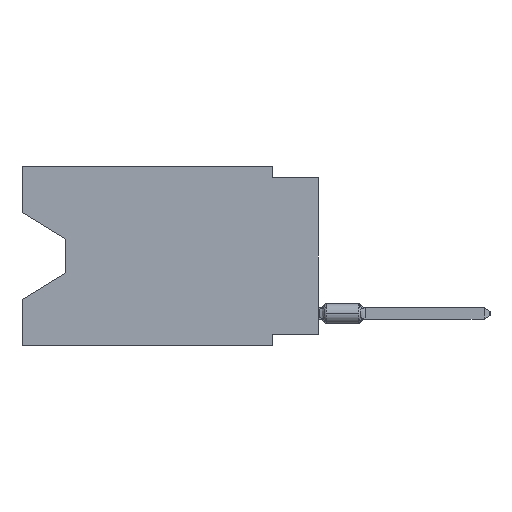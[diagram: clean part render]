
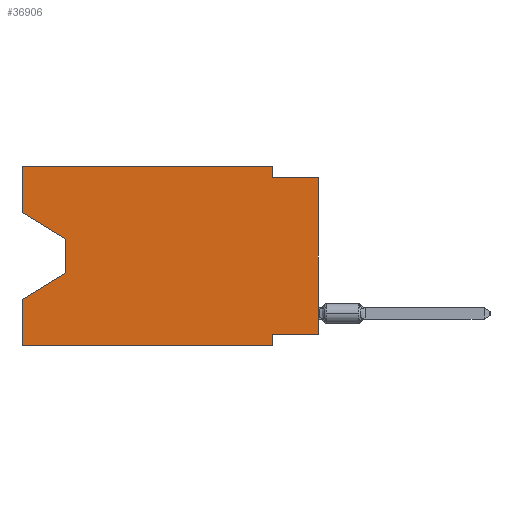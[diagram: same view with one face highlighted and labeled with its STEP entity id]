
A CAD part, left-side view. The second image highlights one B-rep face of the part: STEP entity #36906.
In plain terms, the highlighted planar face has unit normal (-1, 0, 0).
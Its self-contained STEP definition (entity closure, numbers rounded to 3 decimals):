
#1570 = ORIENTED_EDGE ( 'NONE', *, *, #34672, .F. ) ;
#1646 = CARTESIAN_POINT ( 'NONE',  ( 0., 16.383, 0. ) ) ;
#3146 = ORIENTED_EDGE ( 'NONE', *, *, #23481, .T. ) ;
#3249 = VECTOR ( 'NONE', #10510, 1000. ) ;
#3300 = CARTESIAN_POINT ( 'NONE',  ( 0., 16.383, -9.906 ) ) ;
#3720 = EDGE_CURVE ( 'NONE', #20055, #40407, #57582, .T. ) ;
#4301 = VERTEX_POINT ( 'NONE', #23348 ) ;
#4450 = CARTESIAN_POINT ( 'NONE',  ( 0., 0., -0.635 ) ) ;
#5240 = LINE ( 'NONE', #55700, #3249 ) ;
#5429 = CARTESIAN_POINT ( 'NONE',  ( 0., 2.54, -9.906 ) ) ;
#5473 = VECTOR ( 'NONE', #40983, 1000. ) ;
#6020 = VECTOR ( 'NONE', #51335, 1000. ) ;
#6224 = VERTEX_POINT ( 'NONE', #4450 ) ;
#7016 = CARTESIAN_POINT ( 'NONE',  ( 0., 2.54, 0. ) ) ;
#7504 = CARTESIAN_POINT ( 'NONE',  ( 0., 13.97, -5.893 ) ) ;
#8393 = CARTESIAN_POINT ( 'NONE',  ( 0., 2.54, 0. ) ) ;
#9225 = CARTESIAN_POINT ( 'NONE',  ( 0., 16.383, -7.36 ) ) ;
#10033 = FACE_OUTER_BOUND ( 'NONE', #16838, .T. ) ;
#10403 = DIRECTION ( 'NONE',  ( 0., 0., -1. ) ) ;
#10510 = DIRECTION ( 'NONE',  ( 0., 1., 0. ) ) ;
#10766 = EDGE_CURVE ( 'NONE', #26758, #56747, #36832, .T. ) ;
#11138 = PLANE ( 'NONE',  #38106 ) ;
#11255 = EDGE_CURVE ( 'NONE', #62127, #6224, #18677, .T. ) ;
#13391 = LINE ( 'NONE', #7016, #31921 ) ;
#14944 = LINE ( 'NONE', #3300, #43473 ) ;
#14978 = ORIENTED_EDGE ( 'NONE', *, *, #29583, .T. ) ;
#15608 = CARTESIAN_POINT ( 'NONE',  ( 0., 0., -9.271 ) ) ;
#16241 = VECTOR ( 'NONE', #24586, 1000. ) ;
#16386 = VECTOR ( 'NONE', #64615, 1000. ) ;
#16838 = EDGE_LOOP ( 'NONE', ( #51085, #14978, #63160, #18226, #58451, #65640, #35333, #3146, #51564, #34898, #33707, #1570 ) ) ;
#17080 = EDGE_CURVE ( 'NONE', #40627, #57894, #56996, .T. ) ;
#18226 = ORIENTED_EDGE ( 'NONE', *, *, #32633, .F. ) ;
#18677 = LINE ( 'NONE', #41646, #16386 ) ;
#19133 = CARTESIAN_POINT ( 'NONE',  ( 0., 13.97, -4.013 ) ) ;
#19805 = CARTESIAN_POINT ( 'NONE',  ( 0., 16.383, 0. ) ) ;
#20055 = VERTEX_POINT ( 'NONE', #38810 ) ;
#20527 = VECTOR ( 'NONE', #57102, 1000. ) ;
#23348 = CARTESIAN_POINT ( 'NONE',  ( 0., 16.383, -9.906 ) ) ;
#23481 = EDGE_CURVE ( 'NONE', #73886, #6224, #68775, .T. ) ;
#24586 = DIRECTION ( 'NONE',  ( 0., 0., 1. ) ) ;
#24704 = VECTOR ( 'NONE', #47370, 1000. ) ;
#26440 = VECTOR ( 'NONE', #57715, 1000. ) ;
#26758 = VERTEX_POINT ( 'NONE', #62379 ) ;
#29583 = EDGE_CURVE ( 'NONE', #56747, #20055, #70055, .T. ) ;
#29831 = LINE ( 'NONE', #46038, #26440 ) ;
#29864 = LINE ( 'NONE', #1646, #16241 ) ;
#30479 = EDGE_CURVE ( 'NONE', #39617, #62127, #13391, .T. ) ;
#30658 = VECTOR ( 'NONE', #57644, 1000. ) ;
#31921 = VECTOR ( 'NONE', #35970, 1000. ) ;
#32633 = EDGE_CURVE ( 'NONE', #4301, #40407, #42075, .T. ) ;
#33707 = ORIENTED_EDGE ( 'NONE', *, *, #39507, .F. ) ;
#34672 = EDGE_CURVE ( 'NONE', #26758, #59126, #29864, .T. ) ;
#34898 = ORIENTED_EDGE ( 'NONE', *, *, #30479, .F. ) ;
#35333 = ORIENTED_EDGE ( 'NONE', *, *, #70067, .F. ) ;
#35970 = DIRECTION ( 'NONE',  ( 0., 0., -1. ) ) ;
#36832 = LINE ( 'NONE', #42860, #24704 ) ;
#36906 = ADVANCED_FACE ( 'NONE', ( #10033 ), #11138, .F. ) ;
#38106 = AXIS2_PLACEMENT_3D ( 'NONE', #38989, #61964, #10403 ) ;
#38810 = CARTESIAN_POINT ( 'NONE',  ( 0., 13.97, -5.893 ) ) ;
#38989 = CARTESIAN_POINT ( 'NONE',  ( 0., 16.383, 0. ) ) ;
#39507 = EDGE_CURVE ( 'NONE', #59126, #39617, #29831, .T. ) ;
#39617 = VERTEX_POINT ( 'NONE', #8393 ) ;
#40407 = VERTEX_POINT ( 'NONE', #9225 ) ;
#40627 = VERTEX_POINT ( 'NONE', #44940 ) ;
#40875 = CARTESIAN_POINT ( 'NONE',  ( 0., 0., 0. ) ) ;
#40983 = DIRECTION ( 'NONE',  ( 0., 0.855, -0.519 ) ) ;
#41646 = CARTESIAN_POINT ( 'NONE',  ( 0., 0., -0.635 ) ) ;
#42075 = LINE ( 'NONE', #65052, #70453 ) ;
#42860 = CARTESIAN_POINT ( 'NONE',  ( 0., 16.383, -2.546 ) ) ;
#43473 = VECTOR ( 'NONE', #49193, 1000. ) ;
#44940 = CARTESIAN_POINT ( 'NONE',  ( 0., 2.54, -9.271 ) ) ;
#46038 = CARTESIAN_POINT ( 'NONE',  ( 0., 16.383, 0. ) ) ;
#46698 = CARTESIAN_POINT ( 'NONE',  ( 0., 13.97, -4.013 ) ) ;
#47370 = DIRECTION ( 'NONE',  ( 0., -0.855, -0.519 ) ) ;
#48224 = CARTESIAN_POINT ( 'NONE',  ( 0., 2.54, -0.635 ) ) ;
#49193 = DIRECTION ( 'NONE',  ( 0., -1., 0. ) ) ;
#50888 = CARTESIAN_POINT ( 'NONE',  ( 0., 2.54, -9.906 ) ) ;
#51085 = ORIENTED_EDGE ( 'NONE', *, *, #10766, .T. ) ;
#51335 = DIRECTION ( 'NONE',  ( 0., 0., -1. ) ) ;
#51564 = ORIENTED_EDGE ( 'NONE', *, *, #11255, .F. ) ;
#55700 = CARTESIAN_POINT ( 'NONE',  ( 0., 0., -9.271 ) ) ;
#56747 = VERTEX_POINT ( 'NONE', #19133 ) ;
#56996 = LINE ( 'NONE', #5429, #6020 ) ;
#57102 = DIRECTION ( 'NONE',  ( 0., 0., 1. ) ) ;
#57582 = LINE ( 'NONE', #7504, #5473 ) ;
#57644 = DIRECTION ( 'NONE',  ( 0., 0., -1. ) ) ;
#57715 = DIRECTION ( 'NONE',  ( 0., -1., 0. ) ) ;
#57894 = VERTEX_POINT ( 'NONE', #50888 ) ;
#58451 = ORIENTED_EDGE ( 'NONE', *, *, #63494, .T. ) ;
#59126 = VERTEX_POINT ( 'NONE', #19805 ) ;
#59777 = DIRECTION ( 'NONE',  ( 0., 0., 1. ) ) ;
#61964 = DIRECTION ( 'NONE',  ( 1., 0., 0. ) ) ;
#62127 = VERTEX_POINT ( 'NONE', #48224 ) ;
#62379 = CARTESIAN_POINT ( 'NONE',  ( 0., 16.383, -2.546 ) ) ;
#63160 = ORIENTED_EDGE ( 'NONE', *, *, #3720, .T. ) ;
#63494 = EDGE_CURVE ( 'NONE', #4301, #57894, #14944, .T. ) ;
#64615 = DIRECTION ( 'NONE',  ( 0., -1., 0. ) ) ;
#65052 = CARTESIAN_POINT ( 'NONE',  ( 0., 16.383, 0. ) ) ;
#65640 = ORIENTED_EDGE ( 'NONE', *, *, #17080, .F. ) ;
#68775 = LINE ( 'NONE', #40875, #20527 ) ;
#70055 = LINE ( 'NONE', #46698, #30658 ) ;
#70067 = EDGE_CURVE ( 'NONE', #73886, #40627, #5240, .T. ) ;
#70453 = VECTOR ( 'NONE', #59777, 1000. ) ;
#73886 = VERTEX_POINT ( 'NONE', #15608 ) ;
